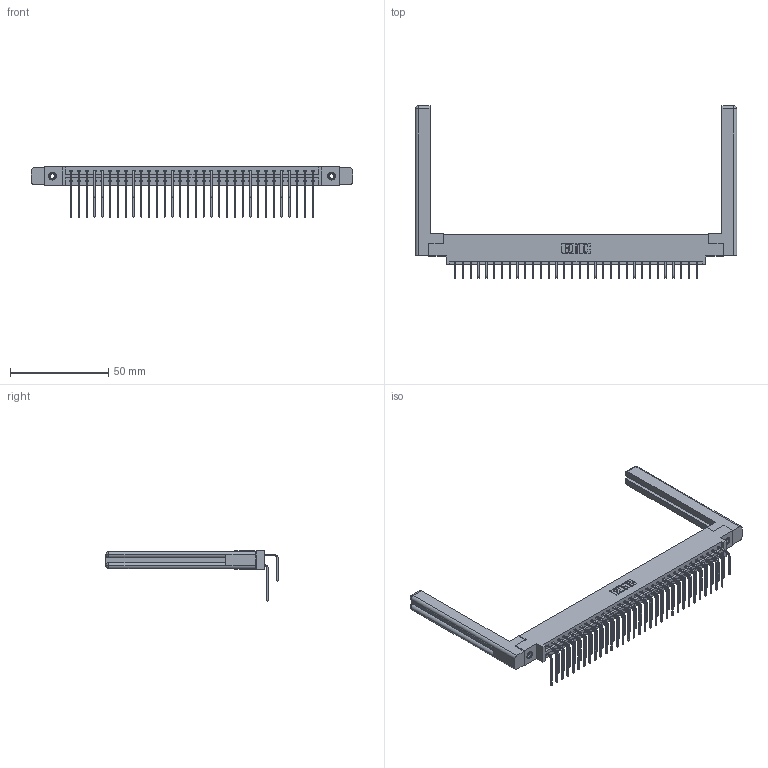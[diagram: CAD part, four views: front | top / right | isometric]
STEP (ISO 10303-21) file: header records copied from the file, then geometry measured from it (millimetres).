
FILE_DESCRIPTION (( 'STEP AP203' ), '1' );
FILE_NAME ('337-064-558-858.STEP', '2019-10-12T00:16:12', ( '' ), ( '' ), 'SwSTEP 2.0', 'SolidWorks 2016', '' );
FILE_SCHEMA (( 'CONFIG_CONTROL_DESIGN' ));
Length unit declared in the file: inch
Products named in the file (6): 337-064-558-858; 337 Part_0.170 Offset - 0.156 Dia-TI; 345-292-001_558 559 Tail - 1; 345-292-001_558 Tail - 2; 307-220-058; 345-250-001_345-250-001-102
Assembly tree (69 placements, depth 2):
  337-064-558-858
    337 Part_0.170 Offset - 0.156 Dia-TI
    345-292-001_558 559 Tail - 1  x32
    345-292-001_558 Tail - 2  x32
    345-250-001_345-250-001-102  x2
    307-220-058  x2
Bounding box: 163.42 x 87.57 x 25.53 mm (x, y, z)
Volume: 24483.8 mm3; surface area: 26515.8 mm2
Topology: 69 solids, 69 shells, 3844 faces, 11365 edges, 7478 vertices
Faces by surface type: plane 2718, cylinder 1102, cone 12, torus 12
Entity records: 30654 total; most frequent: CARTESIAN_POINT 5228, ORIENTED_EDGE 5052, DIRECTION 4462, EDGE_CURVE 2526, LINE 2310, VECTOR 2310, VERTEX_POINT 1674, AXIS2_PLACEMENT_3D 1076
